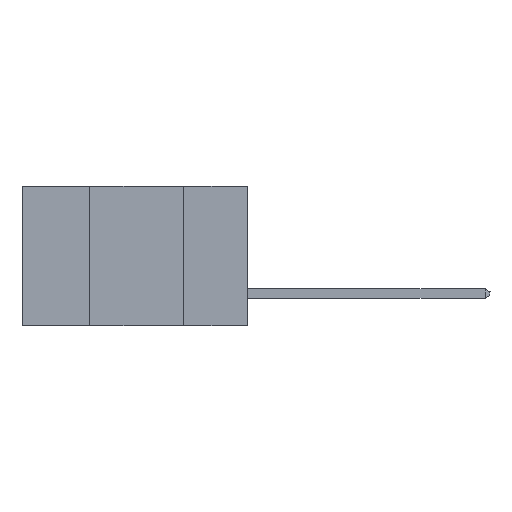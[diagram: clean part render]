
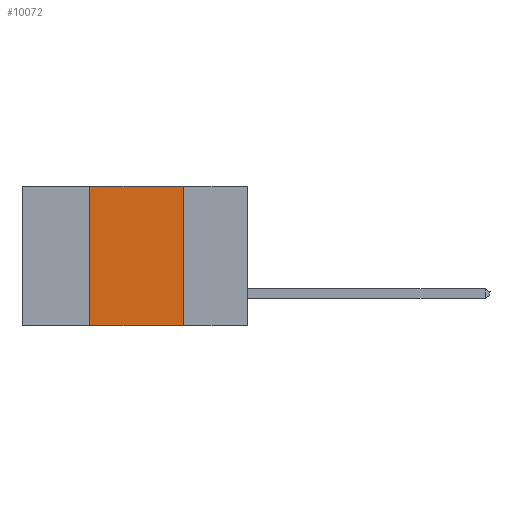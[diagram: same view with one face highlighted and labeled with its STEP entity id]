
A CAD part, left-side view. The second image highlights one B-rep face of the part: STEP entity #10072.
In plain terms, the highlighted planar face has unit normal (-1, 0, 0).
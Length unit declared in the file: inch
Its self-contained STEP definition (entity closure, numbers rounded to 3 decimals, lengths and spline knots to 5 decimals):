
#148 = PLANE ( 'NONE',  #6635 ) ;
#227 = CARTESIAN_POINT ( 'NONE',  ( 0., 0.42, -0.37 ) ) ;
#409 = CARTESIAN_POINT ( 'NONE',  ( 0., 0.17, 0. ) ) ;
#743 = CARTESIAN_POINT ( 'NONE',  ( 0., 0.17, -0.37 ) ) ;
#881 = VERTEX_POINT ( 'NONE', #409 ) ;
#982 = CARTESIAN_POINT ( 'NONE',  ( 0., 0.6, -0.37 ) ) ;
#1149 = ORIENTED_EDGE ( 'NONE', *, *, #1907, .F. ) ;
#1907 = EDGE_CURVE ( 'NONE', #14933, #881, #17560, .T. ) ;
#2616 = ORIENTED_EDGE ( 'NONE', *, *, #10773, .T. ) ;
#2681 = CARTESIAN_POINT ( 'NONE',  ( 0., 0.17, -0.37 ) ) ;
#4805 = EDGE_CURVE ( 'NONE', #881, #13734, #16822, .T. ) ;
#5236 = VERTEX_POINT ( 'NONE', #227 ) ;
#5710 = DIRECTION ( 'NONE',  ( 0., -1., 0. ) ) ;
#5908 = CARTESIAN_POINT ( 'NONE',  ( 0., 0.6, 0. ) ) ;
#6635 = AXIS2_PLACEMENT_3D ( 'NONE', #10465, #10671, #13686 ) ;
#7089 = DIRECTION ( 'NONE',  ( 0., -1., 0. ) ) ;
#7748 = LINE ( 'NONE', #18671, #15964 ) ;
#8074 = CARTESIAN_POINT ( 'NONE',  ( 0., 0.42, 0. ) ) ;
#8787 = DIRECTION ( 'NONE',  ( 0., 0., -1. ) ) ;
#10072 = ADVANCED_FACE ( 'NONE', ( #12082 ), #148, .F. ) ;
#10465 = CARTESIAN_POINT ( 'NONE',  ( 0., 0.6, 0. ) ) ;
#10671 = DIRECTION ( 'NONE',  ( 1., 0., 0. ) ) ;
#10773 = EDGE_CURVE ( 'NONE', #5236, #13734, #19403, .T. ) ;
#11103 = VECTOR ( 'NONE', #8787, 39.37008 ) ;
#11718 = ORIENTED_EDGE ( 'NONE', *, *, #4805, .F. ) ;
#11890 = EDGE_CURVE ( 'NONE', #5236, #14933, #7748, .T. ) ;
#12082 = FACE_OUTER_BOUND ( 'NONE', #16640, .T. ) ;
#13541 = VECTOR ( 'NONE', #5710, 39.37008 ) ;
#13686 = DIRECTION ( 'NONE',  ( 0., 0., -1. ) ) ;
#13713 = ORIENTED_EDGE ( 'NONE', *, *, #11890, .F. ) ;
#13734 = VERTEX_POINT ( 'NONE', #743 ) ;
#13771 = DIRECTION ( 'NONE',  ( 0., 0., 1. ) ) ;
#14933 = VERTEX_POINT ( 'NONE', #8074 ) ;
#15934 = VECTOR ( 'NONE', #7089, 39.37008 ) ;
#15964 = VECTOR ( 'NONE', #13771, 39.37008 ) ;
#16640 = EDGE_LOOP ( 'NONE', ( #11718, #1149, #13713, #2616 ) ) ;
#16822 = LINE ( 'NONE', #2681, #11103 ) ;
#17560 = LINE ( 'NONE', #5908, #13541 ) ;
#18671 = CARTESIAN_POINT ( 'NONE',  ( 0., 0.42, -0.37 ) ) ;
#19403 = LINE ( 'NONE', #982, #15934 ) ;
